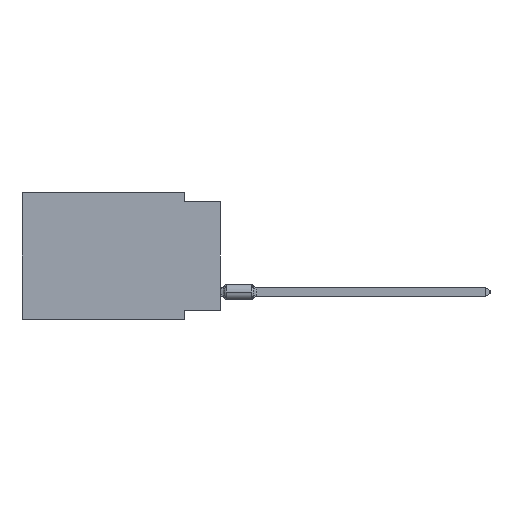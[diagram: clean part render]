
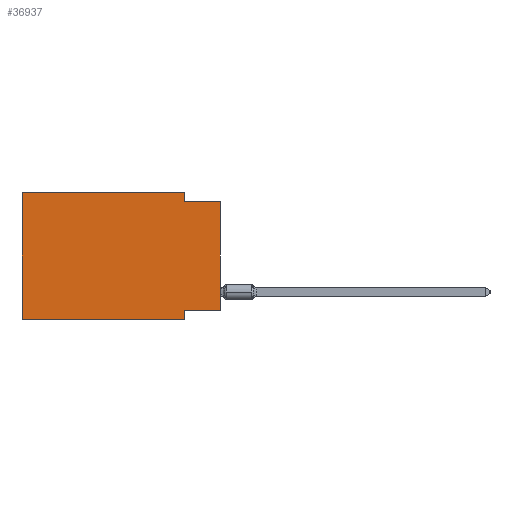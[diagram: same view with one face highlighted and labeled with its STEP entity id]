
A CAD part, left-side view. The second image highlights one B-rep face of the part: STEP entity #36937.
In plain terms, the highlighted planar face has unit normal (-1, 0, 0).
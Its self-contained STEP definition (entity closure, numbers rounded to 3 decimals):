
#898 = EDGE_CURVE ( 'NONE', #34279, #39575, #50530, .T. ) ;
#1042 = DIRECTION ( 'NONE',  ( 0., 0., 1. ) ) ;
#3556 = DIRECTION ( 'NONE',  ( 0., 1., 0. ) ) ;
#4382 = EDGE_CURVE ( 'NONE', #34279, #44023, #57086, .T. ) ;
#4953 = VECTOR ( 'NONE', #5301, 1000. ) ;
#5301 = DIRECTION ( 'NONE',  ( 0., -1., 0. ) ) ;
#5772 = DIRECTION ( 'NONE',  ( 0., 0., 1. ) ) ;
#5975 = CARTESIAN_POINT ( 'NONE',  ( 0., 0., -8.255 ) ) ;
#6077 = VECTOR ( 'NONE', #29145, 1000. ) ;
#8030 = CARTESIAN_POINT ( 'NONE',  ( 0., 2.54, -0.635 ) ) ;
#8210 = ORIENTED_EDGE ( 'NONE', *, *, #34330, .F. ) ;
#9640 = LINE ( 'NONE', #46946, #4953 ) ;
#11430 = VECTOR ( 'NONE', #32203, 1000. ) ;
#11816 = VERTEX_POINT ( 'NONE', #8030 ) ;
#13270 = VERTEX_POINT ( 'NONE', #57691 ) ;
#14696 = LINE ( 'NONE', #37706, #55678 ) ;
#15067 = LINE ( 'NONE', #34027, #36445 ) ;
#15764 = EDGE_CURVE ( 'NONE', #11816, #46917, #9640, .T. ) ;
#16665 = CARTESIAN_POINT ( 'NONE',  ( 0., 2.54, 0. ) ) ;
#17906 = VECTOR ( 'NONE', #41064, 1000. ) ;
#18155 = CARTESIAN_POINT ( 'NONE',  ( 0., 13.97, -8.89 ) ) ;
#18528 = LINE ( 'NONE', #56730, #11430 ) ;
#22084 = CARTESIAN_POINT ( 'NONE',  ( 0., 13.97, 0. ) ) ;
#23462 = DIRECTION ( 'NONE',  ( 0., 0., -1. ) ) ;
#24132 = ORIENTED_EDGE ( 'NONE', *, *, #58948, .F. ) ;
#24727 = VECTOR ( 'NONE', #5772, 1000. ) ;
#24822 = EDGE_LOOP ( 'NONE', ( #36891, #27247, #57002, #24132, #48742, #42864, #39150, #8210 ) ) ;
#27247 = ORIENTED_EDGE ( 'NONE', *, *, #15764, .F. ) ;
#27335 = DIRECTION ( 'NONE',  ( 0., 0., -1. ) ) ;
#27676 = CARTESIAN_POINT ( 'NONE',  ( 0., 13.97, 0. ) ) ;
#29145 = DIRECTION ( 'NONE',  ( 0., -1., 0. ) ) ;
#30202 = EDGE_CURVE ( 'NONE', #13270, #44023, #15067, .T. ) ;
#32203 = DIRECTION ( 'NONE',  ( 0., 0., -1. ) ) ;
#33805 = VERTEX_POINT ( 'NONE', #16665 ) ;
#33837 = VECTOR ( 'NONE', #3556, 1000. ) ;
#34027 = CARTESIAN_POINT ( 'NONE',  ( 0., 2.54, -8.89 ) ) ;
#34279 = VERTEX_POINT ( 'NONE', #18155 ) ;
#34330 = EDGE_CURVE ( 'NONE', #36738, #13270, #46122, .T. ) ;
#34672 = CARTESIAN_POINT ( 'NONE',  ( 0., 2.54, -8.89 ) ) ;
#36059 = PLANE ( 'NONE',  #42903 ) ;
#36102 = EDGE_CURVE ( 'NONE', #36738, #46917, #14696, .T. ) ;
#36445 = VECTOR ( 'NONE', #23462, 1000. ) ;
#36738 = VERTEX_POINT ( 'NONE', #5975 ) ;
#36891 = ORIENTED_EDGE ( 'NONE', *, *, #36102, .T. ) ;
#36937 = ADVANCED_FACE ( 'NONE', ( #44485 ), #36059, .F. ) ;
#37706 = CARTESIAN_POINT ( 'NONE',  ( 0., 0., 0. ) ) ;
#39150 = ORIENTED_EDGE ( 'NONE', *, *, #30202, .F. ) ;
#39575 = VERTEX_POINT ( 'NONE', #48076 ) ;
#41064 = DIRECTION ( 'NONE',  ( 0., -1., 0. ) ) ;
#42660 = EDGE_CURVE ( 'NONE', #33805, #11816, #18528, .T. ) ;
#42864 = ORIENTED_EDGE ( 'NONE', *, *, #4382, .T. ) ;
#42903 = AXIS2_PLACEMENT_3D ( 'NONE', #22084, #59950, #27335 ) ;
#43088 = CARTESIAN_POINT ( 'NONE',  ( 0., 13.97, 0. ) ) ;
#44023 = VERTEX_POINT ( 'NONE', #34672 ) ;
#44485 = FACE_OUTER_BOUND ( 'NONE', #24822, .T. ) ;
#46122 = LINE ( 'NONE', #50150, #33837 ) ;
#46917 = VERTEX_POINT ( 'NONE', #59840 ) ;
#46946 = CARTESIAN_POINT ( 'NONE',  ( 0., 0., -0.635 ) ) ;
#48076 = CARTESIAN_POINT ( 'NONE',  ( 0., 13.97, 0. ) ) ;
#48742 = ORIENTED_EDGE ( 'NONE', *, *, #898, .F. ) ;
#50150 = CARTESIAN_POINT ( 'NONE',  ( 0., 0., -8.255 ) ) ;
#50530 = LINE ( 'NONE', #43088, #24727 ) ;
#55678 = VECTOR ( 'NONE', #1042, 1000. ) ;
#55932 = LINE ( 'NONE', #27676, #17906 ) ;
#56730 = CARTESIAN_POINT ( 'NONE',  ( 0., 2.54, 0. ) ) ;
#57002 = ORIENTED_EDGE ( 'NONE', *, *, #42660, .F. ) ;
#57086 = LINE ( 'NONE', #61123, #6077 ) ;
#57691 = CARTESIAN_POINT ( 'NONE',  ( 0., 2.54, -8.255 ) ) ;
#58948 = EDGE_CURVE ( 'NONE', #39575, #33805, #55932, .T. ) ;
#59840 = CARTESIAN_POINT ( 'NONE',  ( 0., 0., -0.635 ) ) ;
#59950 = DIRECTION ( 'NONE',  ( 1., 0., 0. ) ) ;
#61123 = CARTESIAN_POINT ( 'NONE',  ( 0., 13.97, -8.89 ) ) ;
